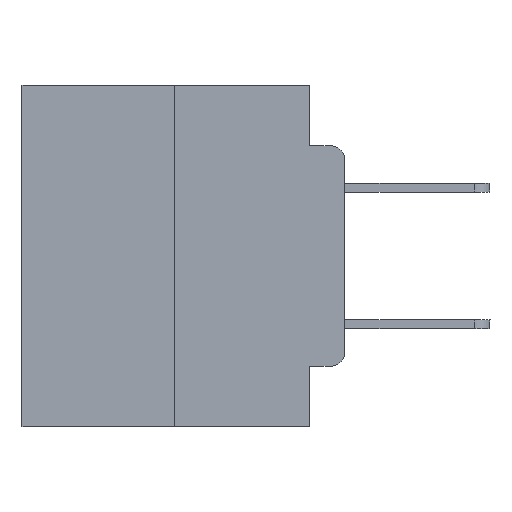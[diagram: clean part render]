
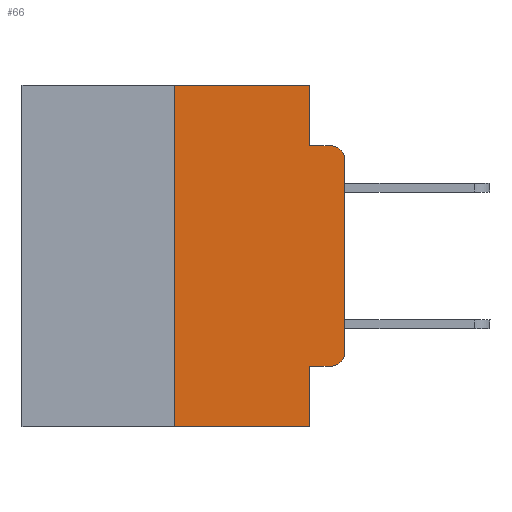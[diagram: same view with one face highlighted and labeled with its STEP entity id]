
A CAD part, left-side view. The second image highlights one B-rep face of the part: STEP entity #66.
In plain terms, the highlighted planar face has unit normal (-1, 0, 0).
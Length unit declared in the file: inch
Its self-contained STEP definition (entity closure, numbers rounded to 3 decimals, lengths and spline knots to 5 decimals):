
#66 = ADVANCED_FACE ( 'NONE', ( #8878 ), #8731, .F. ) ;
#151 = DIRECTION ( 'NONE',  ( 0., -1., 0. ) ) ;
#215 = LINE ( 'NONE', #12985, #2032 ) ;
#289 = CIRCLE ( 'NONE', #24054, 0.02 ) ;
#456 = CARTESIAN_POINT ( 'NONE',  ( 0., 0.473, -0.5 ) ) ;
#659 = DIRECTION ( 'NONE',  ( -1., 0., 0. ) ) ;
#854 = CARTESIAN_POINT ( 'NONE',  ( 0., 0.02, -0.4115 ) ) ;
#904 = VERTEX_POINT ( 'NONE', #9804 ) ;
#923 = CARTESIAN_POINT ( 'NONE',  ( 0., 0.051, 0. ) ) ;
#936 = CARTESIAN_POINT ( 'NONE',  ( 0., 0.25, 0. ) ) ;
#1152 = EDGE_CURVE ( 'NONE', #18230, #11053, #289, .T. ) ;
#1974 = DIRECTION ( 'NONE',  ( 0., -1., 0. ) ) ;
#2032 = VECTOR ( 'NONE', #10894, 39.37008 ) ;
#2980 = DIRECTION ( 'NONE',  ( 0., -1., 0. ) ) ;
#4394 = CARTESIAN_POINT ( 'NONE',  ( 0., 0.473, 0. ) ) ;
#4465 = CARTESIAN_POINT ( 'NONE',  ( 0., 0.02, -0.0885 ) ) ;
#4526 = VERTEX_POINT ( 'NONE', #16315 ) ;
#4666 = ORIENTED_EDGE ( 'NONE', *, *, #13434, .T. ) ;
#4833 = CARTESIAN_POINT ( 'NONE',  ( 0., 0.051, 0. ) ) ;
#4843 = CARTESIAN_POINT ( 'NONE',  ( 0., 0.051, 0. ) ) ;
#5622 = VECTOR ( 'NONE', #151, 39.37008 ) ;
#6108 = VECTOR ( 'NONE', #19577, 39.37008 ) ;
#6190 = ORIENTED_EDGE ( 'NONE', *, *, #1152, .T. ) ;
#6631 = DIRECTION ( 'NONE',  ( 0., 0., -1. ) ) ;
#7724 = VECTOR ( 'NONE', #11892, 39.37008 ) ;
#7964 = VERTEX_POINT ( 'NONE', #923 ) ;
#8084 = ORIENTED_EDGE ( 'NONE', *, *, #22825, .T. ) ;
#8731 = PLANE ( 'NONE',  #18186 ) ;
#8802 = EDGE_CURVE ( 'NONE', #11219, #7964, #11372, .T. ) ;
#8878 = FACE_OUTER_BOUND ( 'NONE', #16652, .T. ) ;
#9221 = ORIENTED_EDGE ( 'NONE', *, *, #19991, .T. ) ;
#9332 = VECTOR ( 'NONE', #2980, 39.37008 ) ;
#9804 = CARTESIAN_POINT ( 'NONE',  ( 0., 0.051, -0.4115 ) ) ;
#10250 = CARTESIAN_POINT ( 'NONE',  ( 0., 0.051, -0.4115 ) ) ;
#10397 = VECTOR ( 'NONE', #20100, 39.37008 ) ;
#10500 = ORIENTED_EDGE ( 'NONE', *, *, #25762, .F. ) ;
#10894 = DIRECTION ( 'NONE',  ( 0., 0., 1. ) ) ;
#11053 = VERTEX_POINT ( 'NONE', #4465 ) ;
#11148 = VECTOR ( 'NONE', #1974, 39.37008 ) ;
#11219 = VERTEX_POINT ( 'NONE', #936 ) ;
#11372 = LINE ( 'NONE', #21518, #5622 ) ;
#11892 = DIRECTION ( 'NONE',  ( 0., -1., 0. ) ) ;
#12241 = AXIS2_PLACEMENT_3D ( 'NONE', #23042, #16709, #16429 ) ;
#12304 = VERTEX_POINT ( 'NONE', #14407 ) ;
#12655 = DIRECTION ( 'NONE',  ( 1., 0., 0. ) ) ;
#12816 = VECTOR ( 'NONE', #15607, 39.37008 ) ;
#12985 = CARTESIAN_POINT ( 'NONE',  ( 0., 0.25, 0. ) ) ;
#13434 = EDGE_CURVE ( 'NONE', #16946, #4526, #19974, .T. ) ;
#13702 = CARTESIAN_POINT ( 'NONE',  ( 0., 0.02, -0.1085 ) ) ;
#13804 = EDGE_CURVE ( 'NONE', #904, #18947, #27570, .T. ) ;
#14407 = CARTESIAN_POINT ( 'NONE',  ( 0., 0., -0.3915 ) ) ;
#15442 = ORIENTED_EDGE ( 'NONE', *, *, #27711, .F. ) ;
#15565 = ORIENTED_EDGE ( 'NONE', *, *, #13804, .T. ) ;
#15607 = DIRECTION ( 'NONE',  ( 0., 0., -1. ) ) ;
#15818 = CIRCLE ( 'NONE', #12241, 0.02 ) ;
#16151 = CARTESIAN_POINT ( 'NONE',  ( 0., 0., 0. ) ) ;
#16315 = CARTESIAN_POINT ( 'NONE',  ( 0., 0.051, -0.5 ) ) ;
#16429 = DIRECTION ( 'NONE',  ( 0., 0., -1. ) ) ;
#16652 = EDGE_LOOP ( 'NONE', ( #9221, #6190, #21247, #15442, #22903, #18369, #4666, #10500, #15565, #8084 ) ) ;
#16709 = DIRECTION ( 'NONE',  ( -1., 0., 0. ) ) ;
#16946 = VERTEX_POINT ( 'NONE', #21890 ) ;
#18081 = LINE ( 'NONE', #26971, #7724 ) ;
#18186 = AXIS2_PLACEMENT_3D ( 'NONE', #4394, #12655, #6631 ) ;
#18230 = VERTEX_POINT ( 'NONE', #26270 ) ;
#18369 = ORIENTED_EDGE ( 'NONE', *, *, #25195, .F. ) ;
#18947 = VERTEX_POINT ( 'NONE', #854 ) ;
#19577 = DIRECTION ( 'NONE',  ( 0., 0., -1. ) ) ;
#19739 = CARTESIAN_POINT ( 'NONE',  ( 0., 0.051, -0.0885 ) ) ;
#19974 = LINE ( 'NONE', #456, #9332 ) ;
#19991 = EDGE_CURVE ( 'NONE', #12304, #18230, #20391, .T. ) ;
#20100 = DIRECTION ( 'NONE',  ( 0., 0., 1. ) ) ;
#20391 = LINE ( 'NONE', #16151, #10397 ) ;
#20513 = EDGE_CURVE ( 'NONE', #27222, #11053, #18081, .T. ) ;
#21247 = ORIENTED_EDGE ( 'NONE', *, *, #20513, .F. ) ;
#21518 = CARTESIAN_POINT ( 'NONE',  ( 0., 0.473, 0. ) ) ;
#21890 = CARTESIAN_POINT ( 'NONE',  ( 0., 0.25, -0.5 ) ) ;
#22008 = DIRECTION ( 'NONE',  ( 0., 0., -1. ) ) ;
#22825 = EDGE_CURVE ( 'NONE', #18947, #12304, #15818, .T. ) ;
#22903 = ORIENTED_EDGE ( 'NONE', *, *, #8802, .F. ) ;
#23042 = CARTESIAN_POINT ( 'NONE',  ( 0., 0.02, -0.3915 ) ) ;
#23910 = LINE ( 'NONE', #4833, #12816 ) ;
#24054 = AXIS2_PLACEMENT_3D ( 'NONE', #13702, #659, #22008 ) ;
#25195 = EDGE_CURVE ( 'NONE', #16946, #11219, #215, .T. ) ;
#25762 = EDGE_CURVE ( 'NONE', #904, #4526, #26056, .T. ) ;
#26056 = LINE ( 'NONE', #4843, #6108 ) ;
#26270 = CARTESIAN_POINT ( 'NONE',  ( 0., 0., -0.1085 ) ) ;
#26971 = CARTESIAN_POINT ( 'NONE',  ( 0., 0.051, -0.0885 ) ) ;
#27222 = VERTEX_POINT ( 'NONE', #19739 ) ;
#27570 = LINE ( 'NONE', #10250, #11148 ) ;
#27711 = EDGE_CURVE ( 'NONE', #7964, #27222, #23910, .T. ) ;
